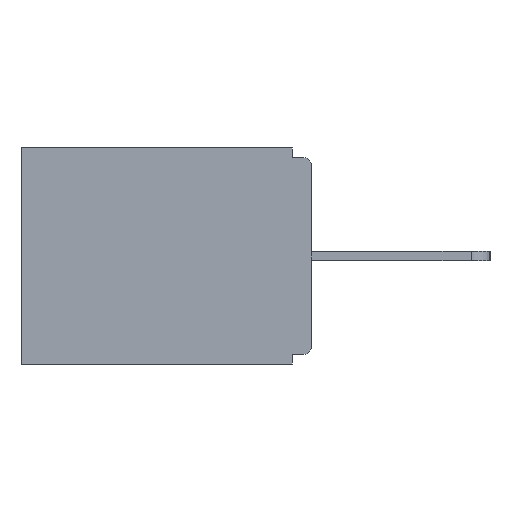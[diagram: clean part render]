
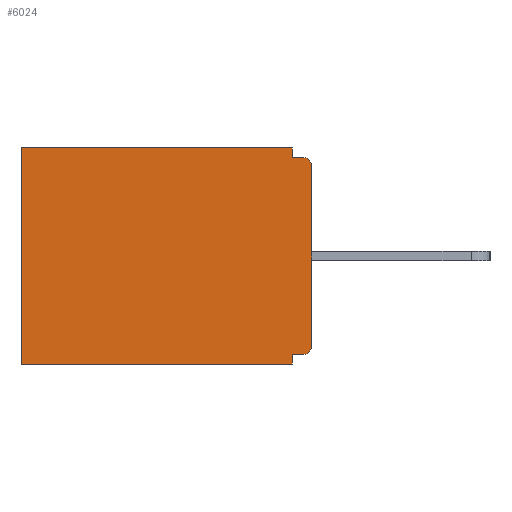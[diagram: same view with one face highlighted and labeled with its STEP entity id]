
A CAD part, left-side view. The second image highlights one B-rep face of the part: STEP entity #6024.
In plain terms, the highlighted planar face has unit normal (-1, 0, 0).
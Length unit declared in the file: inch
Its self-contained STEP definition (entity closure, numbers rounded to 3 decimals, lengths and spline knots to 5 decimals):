
#171 = VERTEX_POINT ( 'NONE', #12377 ) ;
#321 = ORIENTED_EDGE ( 'NONE', *, *, #10879, .F. ) ;
#496 = PLANE ( 'NONE',  #8390 ) ;
#516 = ORIENTED_EDGE ( 'NONE', *, *, #11309, .T. ) ;
#569 = VERTEX_POINT ( 'NONE', #3150 ) ;
#761 = CARTESIAN_POINT ( 'NONE',  ( 0.298, 0., -0.343 ) ) ;
#824 = DIRECTION ( 'NONE',  ( -1., 0., 0. ) ) ;
#1007 = VERTEX_POINT ( 'NONE', #2676 ) ;
#1106 = ORIENTED_EDGE ( 'NONE', *, *, #7103, .F. ) ;
#1542 = CARTESIAN_POINT ( 'NONE',  ( 0.298, 0.015, -0.328 ) ) ;
#1572 = EDGE_CURVE ( 'NONE', #13963, #4232, #2873, .T. ) ;
#1613 = VECTOR ( 'NONE', #6336, 39.37008 ) ;
#2290 = DIRECTION ( 'NONE',  ( 0., 0., -1. ) ) ;
#2492 = ORIENTED_EDGE ( 'NONE', *, *, #1572, .F. ) ;
#2676 = CARTESIAN_POINT ( 'NONE',  ( 0.298, 0.031, -0.015 ) ) ;
#2873 = LINE ( 'NONE', #7287, #7956 ) ;
#3150 = CARTESIAN_POINT ( 'NONE',  ( 0.298, 0., -0.313 ) ) ;
#3990 = ORIENTED_EDGE ( 'NONE', *, *, #13617, .F. ) ;
#4157 = VERTEX_POINT ( 'NONE', #8587 ) ;
#4158 = ORIENTED_EDGE ( 'NONE', *, *, #8078, .F. ) ;
#4232 = VERTEX_POINT ( 'NONE', #9609 ) ;
#4620 = CARTESIAN_POINT ( 'NONE',  ( 0.298, 0.46, 0. ) ) ;
#4894 = EDGE_CURVE ( 'NONE', #4157, #11916, #12911, .T. ) ;
#5266 = VECTOR ( 'NONE', #7126, 39.37008 ) ;
#5329 = ORIENTED_EDGE ( 'NONE', *, *, #4894, .F. ) ;
#5438 = CARTESIAN_POINT ( 'NONE',  ( 0.298, 0.015, -0.03 ) ) ;
#5473 = LINE ( 'NONE', #11698, #13553 ) ;
#5494 = CARTESIAN_POINT ( 'NONE',  ( 0.298, 0.015, -0.015 ) ) ;
#5502 = ORIENTED_EDGE ( 'NONE', *, *, #8473, .T. ) ;
#5698 = VECTOR ( 'NONE', #2290, 39.37008 ) ;
#5706 = DIRECTION ( 'NONE',  ( 0., 1., 0. ) ) ;
#5723 = VECTOR ( 'NONE', #11137, 39.37008 ) ;
#5849 = DIRECTION ( 'NONE',  ( 0., 0., -1. ) ) ;
#6024 = ADVANCED_FACE ( 'NONE', ( #10406 ), #496, .F. ) ;
#6336 = DIRECTION ( 'NONE',  ( 0., 0., -1. ) ) ;
#6390 = DIRECTION ( 'NONE',  ( 1., 0., 0. ) ) ;
#6425 = VECTOR ( 'NONE', #5706, 39.37008 ) ;
#6448 = DIRECTION ( 'NONE',  ( 0., 0., -1. ) ) ;
#7103 = EDGE_CURVE ( 'NONE', #9262, #1007, #7690, .T. ) ;
#7126 = DIRECTION ( 'NONE',  ( 0., 0., -1. ) ) ;
#7221 = ORIENTED_EDGE ( 'NONE', *, *, #11770, .T. ) ;
#7243 = VECTOR ( 'NONE', #7717, 39.37008 ) ;
#7287 = CARTESIAN_POINT ( 'NONE',  ( 0.298, 0., -0.328 ) ) ;
#7461 = CIRCLE ( 'NONE', #9142, 0.015 ) ;
#7491 = LINE ( 'NONE', #12719, #1613 ) ;
#7502 = CARTESIAN_POINT ( 'NONE',  ( 0.298, 0.015, -0.313 ) ) ;
#7627 = CARTESIAN_POINT ( 'NONE',  ( 0.298, 0.031, 0. ) ) ;
#7690 = LINE ( 'NONE', #9308, #5266 ) ;
#7717 = DIRECTION ( 'NONE',  ( 0., 1., 0. ) ) ;
#7956 = VECTOR ( 'NONE', #11195, 39.37008 ) ;
#8078 = EDGE_CURVE ( 'NONE', #4232, #4157, #13790, .T. ) ;
#8175 = VERTEX_POINT ( 'NONE', #5494 ) ;
#8390 = AXIS2_PLACEMENT_3D ( 'NONE', #11947, #6390, #5849 ) ;
#8473 = EDGE_CURVE ( 'NONE', #171, #8175, #10381, .T. ) ;
#8578 = DIRECTION ( 'NONE',  ( 0., 0., -1. ) ) ;
#8587 = CARTESIAN_POINT ( 'NONE',  ( 0.298, 0.031, -0.343 ) ) ;
#8633 = ORIENTED_EDGE ( 'NONE', *, *, #13128, .T. ) ;
#8810 = LINE ( 'NONE', #4620, #5698 ) ;
#9142 = AXIS2_PLACEMENT_3D ( 'NONE', #7502, #824, #8578 ) ;
#9262 = VERTEX_POINT ( 'NONE', #7627 ) ;
#9308 = CARTESIAN_POINT ( 'NONE',  ( 0.298, 0.031, -0.343 ) ) ;
#9358 = EDGE_LOOP ( 'NONE', ( #5502, #3990, #1106, #8633, #516, #5329, #4158, #2492, #7221, #321 ) ) ;
#9609 = CARTESIAN_POINT ( 'NONE',  ( 0.298, 0.031, -0.328 ) ) ;
#9814 = CARTESIAN_POINT ( 'NONE',  ( 0.298, 0.46, -0.343 ) ) ;
#10381 = CIRCLE ( 'NONE', #12586, 0.015 ) ;
#10406 = FACE_OUTER_BOUND ( 'NONE', #9358, .T. ) ;
#10676 = DIRECTION ( 'NONE',  ( 0., -1., 0. ) ) ;
#10879 = EDGE_CURVE ( 'NONE', #171, #569, #7491, .T. ) ;
#11137 = DIRECTION ( 'NONE',  ( 0., 0., -1. ) ) ;
#11195 = DIRECTION ( 'NONE',  ( 0., 1., 0. ) ) ;
#11246 = CARTESIAN_POINT ( 'NONE',  ( 0.298, 0.46, 0. ) ) ;
#11309 = EDGE_CURVE ( 'NONE', #12693, #11916, #8810, .T. ) ;
#11698 = CARTESIAN_POINT ( 'NONE',  ( 0.298, 0., -0.015 ) ) ;
#11746 = LINE ( 'NONE', #12038, #6425 ) ;
#11770 = EDGE_CURVE ( 'NONE', #13963, #569, #7461, .T. ) ;
#11916 = VERTEX_POINT ( 'NONE', #9814 ) ;
#11947 = CARTESIAN_POINT ( 'NONE',  ( 0.298, 0., 0. ) ) ;
#12038 = CARTESIAN_POINT ( 'NONE',  ( 0.298, 0., 0. ) ) ;
#12377 = CARTESIAN_POINT ( 'NONE',  ( 0.298, 0., -0.03 ) ) ;
#12586 = AXIS2_PLACEMENT_3D ( 'NONE', #5438, #12822, #6448 ) ;
#12692 = CARTESIAN_POINT ( 'NONE',  ( 0.298, 0.031, -0.343 ) ) ;
#12693 = VERTEX_POINT ( 'NONE', #11246 ) ;
#12719 = CARTESIAN_POINT ( 'NONE',  ( 0.298, 0., 0. ) ) ;
#12822 = DIRECTION ( 'NONE',  ( -1., 0., 0. ) ) ;
#12911 = LINE ( 'NONE', #761, #7243 ) ;
#13128 = EDGE_CURVE ( 'NONE', #9262, #12693, #11746, .T. ) ;
#13553 = VECTOR ( 'NONE', #10676, 39.37008 ) ;
#13617 = EDGE_CURVE ( 'NONE', #1007, #8175, #5473, .T. ) ;
#13790 = LINE ( 'NONE', #12692, #5723 ) ;
#13963 = VERTEX_POINT ( 'NONE', #1542 ) ;
